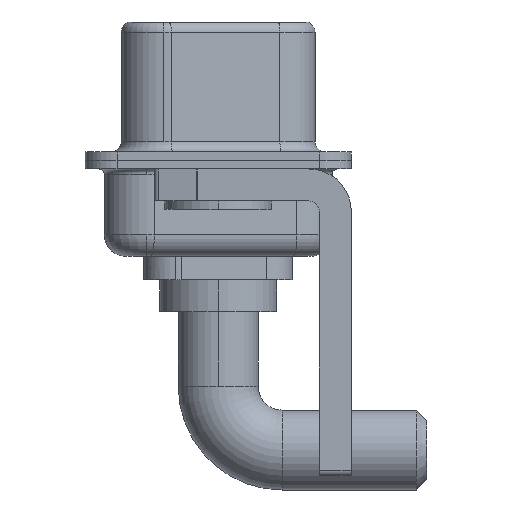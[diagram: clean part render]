
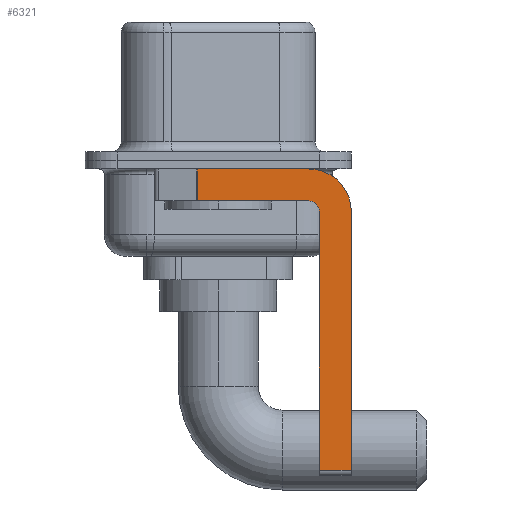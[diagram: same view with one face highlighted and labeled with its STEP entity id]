
A CAD part, left-side view. The second image highlights one B-rep face of the part: STEP entity #6321.
In plain terms, the highlighted planar face has unit normal (-1, 0, 0).
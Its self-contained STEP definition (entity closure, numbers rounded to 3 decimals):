
#196 = DIRECTION ( 'NONE',  ( 1., 0., 0. ) ) ;
#437 = CARTESIAN_POINT ( 'NONE',  ( -2.9, -6.25, -14.55 ) ) ;
#465 = CARTESIAN_POINT ( 'NONE',  ( -2.9, -4.75, -14.55 ) ) ;
#883 = CARTESIAN_POINT ( 'NONE',  ( -2.9, -4.25, -1.9 ) ) ;
#1236 = ORIENTED_EDGE ( 'NONE', *, *, #14373, .F. ) ;
#1631 = EDGE_CURVE ( 'NONE', #12865, #13221, #2365, .T. ) ;
#1837 = EDGE_CURVE ( 'NONE', #8945, #8989, #2182, .T. ) ;
#1890 = AXIS2_PLACEMENT_3D ( 'NONE', #14907, #10285, #4481 ) ;
#2182 = LINE ( 'NONE', #13766, #14195 ) ;
#2253 = ORIENTED_EDGE ( 'NONE', *, *, #4558, .F. ) ;
#2361 = AXIS2_PLACEMENT_3D ( 'NONE', #7664, #10095, #2990 ) ;
#2365 = LINE ( 'NONE', #6032, #4625 ) ;
#2429 = PLANE ( 'NONE',  #6377 ) ;
#2849 = ORIENTED_EDGE ( 'NONE', *, *, #4576, .F. ) ;
#2972 = DIRECTION ( 'NONE',  ( 0., -1., 0. ) ) ;
#2990 = DIRECTION ( 'NONE',  ( 0., 0., -1. ) ) ;
#3238 = LINE ( 'NONE', #11202, #5960 ) ;
#3516 = EDGE_CURVE ( 'NONE', #8945, #10913, #8713, .T. ) ;
#3731 = ORIENTED_EDGE ( 'NONE', *, *, #6710, .F. ) ;
#3836 = CIRCLE ( 'NONE', #2361, 2. ) ;
#4393 = DIRECTION ( 'NONE',  ( 0., -1., 0. ) ) ;
#4481 = DIRECTION ( 'NONE',  ( 0., 0., 1. ) ) ;
#4558 = EDGE_CURVE ( 'NONE', #12865, #7123, #5384, .T. ) ;
#4576 = EDGE_CURVE ( 'NONE', #9478, #10913, #3238, .T. ) ;
#4593 = DIRECTION ( 'NONE',  ( 0., 0., -1. ) ) ;
#4625 = VECTOR ( 'NONE', #4593, 1000. ) ;
#5352 = CARTESIAN_POINT ( 'NONE',  ( -2.9, -4.25, -1.9 ) ) ;
#5384 = LINE ( 'NONE', #6525, #13557 ) ;
#5960 = VECTOR ( 'NONE', #7908, 1000. ) ;
#6032 = CARTESIAN_POINT ( 'NONE',  ( -2.9, 0.978, -1.9 ) ) ;
#6321 = ADVANCED_FACE ( 'NONE', ( #10534 ), #2429, .F. ) ;
#6377 = AXIS2_PLACEMENT_3D ( 'NONE', #11839, #196, #14088 ) ;
#6525 = CARTESIAN_POINT ( 'NONE',  ( -2.9, 3., -0.4 ) ) ;
#6710 = EDGE_CURVE ( 'NONE', #8989, #14838, #8491, .T. ) ;
#7123 = VERTEX_POINT ( 'NONE', #14729 ) ;
#7664 = CARTESIAN_POINT ( 'NONE',  ( -2.9, -4.25, -2.4 ) ) ;
#7908 = DIRECTION ( 'NONE',  ( 0., 0., -1. ) ) ;
#8169 = CARTESIAN_POINT ( 'NONE',  ( -2.9, 0.978, -1.9 ) ) ;
#8491 = CIRCLE ( 'NONE', #1890, 0.5 ) ;
#8713 = LINE ( 'NONE', #14407, #9587 ) ;
#8860 = LINE ( 'NONE', #5352, #14857 ) ;
#8945 = VERTEX_POINT ( 'NONE', #465 ) ;
#8989 = VERTEX_POINT ( 'NONE', #9800 ) ;
#9267 = ORIENTED_EDGE ( 'NONE', *, *, #1631, .T. ) ;
#9478 = VERTEX_POINT ( 'NONE', #13023 ) ;
#9587 = VECTOR ( 'NONE', #2972, 1000. ) ;
#9800 = CARTESIAN_POINT ( 'NONE',  ( -2.9, -4.75, -2.4 ) ) ;
#10095 = DIRECTION ( 'NONE',  ( 1., 0., 0. ) ) ;
#10285 = DIRECTION ( 'NONE',  ( -1., 0., 0. ) ) ;
#10534 = FACE_OUTER_BOUND ( 'NONE', #12693, .T. ) ;
#10913 = VERTEX_POINT ( 'NONE', #437 ) ;
#11202 = CARTESIAN_POINT ( 'NONE',  ( -2.9, -6.25, -2.4 ) ) ;
#11514 = ORIENTED_EDGE ( 'NONE', *, *, #1837, .F. ) ;
#11839 = CARTESIAN_POINT ( 'NONE',  ( -2.9, -4.25, -2.4 ) ) ;
#12693 = EDGE_LOOP ( 'NONE', ( #2253, #9267, #13936, #3731, #11514, #14620, #2849, #1236 ) ) ;
#12865 = VERTEX_POINT ( 'NONE', #13573 ) ;
#13023 = CARTESIAN_POINT ( 'NONE',  ( -2.9, -6.25, -2.4 ) ) ;
#13209 = EDGE_CURVE ( 'NONE', #14838, #13221, #8860, .T. ) ;
#13221 = VERTEX_POINT ( 'NONE', #8169 ) ;
#13556 = DIRECTION ( 'NONE',  ( 0., 1., 0. ) ) ;
#13557 = VECTOR ( 'NONE', #4393, 1000. ) ;
#13573 = CARTESIAN_POINT ( 'NONE',  ( -2.9, 0.978, -0.4 ) ) ;
#13766 = CARTESIAN_POINT ( 'NONE',  ( -2.9, -4.75, -14.8 ) ) ;
#13936 = ORIENTED_EDGE ( 'NONE', *, *, #13209, .F. ) ;
#14088 = DIRECTION ( 'NONE',  ( 0., 0., -1. ) ) ;
#14195 = VECTOR ( 'NONE', #14980, 1000. ) ;
#14373 = EDGE_CURVE ( 'NONE', #7123, #9478, #3836, .T. ) ;
#14407 = CARTESIAN_POINT ( 'NONE',  ( -2.9, -4.25, -14.55 ) ) ;
#14620 = ORIENTED_EDGE ( 'NONE', *, *, #3516, .T. ) ;
#14729 = CARTESIAN_POINT ( 'NONE',  ( -2.9, -4.25, -0.4 ) ) ;
#14838 = VERTEX_POINT ( 'NONE', #883 ) ;
#14857 = VECTOR ( 'NONE', #13556, 1000. ) ;
#14907 = CARTESIAN_POINT ( 'NONE',  ( -2.9, -4.25, -2.4 ) ) ;
#14980 = DIRECTION ( 'NONE',  ( 0., 0., 1. ) ) ;
